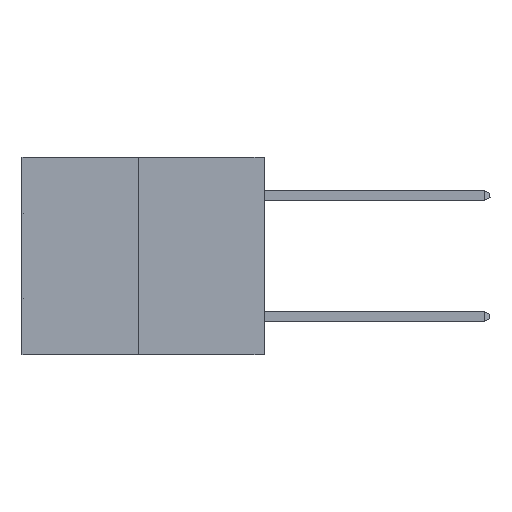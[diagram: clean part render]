
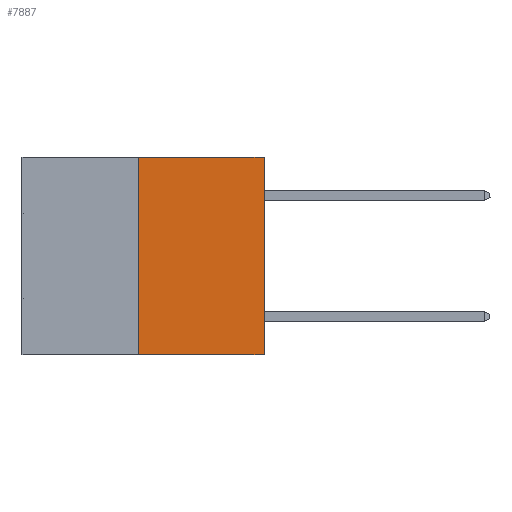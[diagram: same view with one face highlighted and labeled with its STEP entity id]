
A CAD part, left-side view. The second image highlights one B-rep face of the part: STEP entity #7887.
In plain terms, the highlighted planar face has unit normal (-1, 0, 0).
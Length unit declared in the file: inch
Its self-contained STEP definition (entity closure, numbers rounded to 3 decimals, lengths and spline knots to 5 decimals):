
#1921 = EDGE_CURVE ( 'NONE', #18268, #29433, #10328, .T. ) ;
#2554 = CARTESIAN_POINT ( 'NONE',  ( 0., 0., 0. ) ) ;
#2980 = DIRECTION ( 'NONE',  ( 0., 0., 1. ) ) ;
#3670 = DIRECTION ( 'NONE',  ( 0., -1., 0. ) ) ;
#4888 = ORIENTED_EDGE ( 'NONE', *, *, #13954, .T. ) ;
#4945 = CARTESIAN_POINT ( 'NONE',  ( 0., 0.312, -0.49 ) ) ;
#5951 = PLANE ( 'NONE',  #12810 ) ;
#7887 = ADVANCED_FACE ( 'NONE', ( #23895 ), #5951, .F. ) ;
#9751 = EDGE_CURVE ( 'NONE', #18268, #18713, #15423, .T. ) ;
#10323 = VECTOR ( 'NONE', #2980, 39.37008 ) ;
#10328 = LINE ( 'NONE', #31625, #14731 ) ;
#12334 = DIRECTION ( 'NONE',  ( 0., -1., 0. ) ) ;
#12436 = ORIENTED_EDGE ( 'NONE', *, *, #17528, .F. ) ;
#12649 = CARTESIAN_POINT ( 'NONE',  ( 0., 0., -0.49 ) ) ;
#12810 = AXIS2_PLACEMENT_3D ( 'NONE', #28493, #13309, #20948 ) ;
#13309 = DIRECTION ( 'NONE',  ( 1., 0., 0. ) ) ;
#13436 = VECTOR ( 'NONE', #12334, 39.37008 ) ;
#13954 = EDGE_CURVE ( 'NONE', #18713, #21455, #17496, .T. ) ;
#13986 = DIRECTION ( 'NONE',  ( 0., 0., 1. ) ) ;
#14731 = VECTOR ( 'NONE', #13986, 39.37008 ) ;
#14854 = CARTESIAN_POINT ( 'NONE',  ( 0., 0.312, 0. ) ) ;
#15423 = LINE ( 'NONE', #32691, #13436 ) ;
#15874 = EDGE_LOOP ( 'NONE', ( #31179, #31036, #4888, #12436 ) ) ;
#16095 = VECTOR ( 'NONE', #3670, 39.37008 ) ;
#16602 = CARTESIAN_POINT ( 'NONE',  ( 0., 0., 0. ) ) ;
#17496 = LINE ( 'NONE', #2554, #10323 ) ;
#17528 = EDGE_CURVE ( 'NONE', #29433, #21455, #24420, .T. ) ;
#18268 = VERTEX_POINT ( 'NONE', #4945 ) ;
#18713 = VERTEX_POINT ( 'NONE', #12649 ) ;
#20948 = DIRECTION ( 'NONE',  ( 0., 0., -1. ) ) ;
#21203 = CARTESIAN_POINT ( 'NONE',  ( 0., 0.6, 0. ) ) ;
#21455 = VERTEX_POINT ( 'NONE', #16602 ) ;
#23895 = FACE_OUTER_BOUND ( 'NONE', #15874, .T. ) ;
#24420 = LINE ( 'NONE', #21203, #16095 ) ;
#28493 = CARTESIAN_POINT ( 'NONE',  ( 0., 0.6, 0. ) ) ;
#29433 = VERTEX_POINT ( 'NONE', #14854 ) ;
#31036 = ORIENTED_EDGE ( 'NONE', *, *, #9751, .T. ) ;
#31179 = ORIENTED_EDGE ( 'NONE', *, *, #1921, .F. ) ;
#31625 = CARTESIAN_POINT ( 'NONE',  ( 0., 0.312, -0.49 ) ) ;
#32691 = CARTESIAN_POINT ( 'NONE',  ( 0., 0.6, -0.49 ) ) ;
